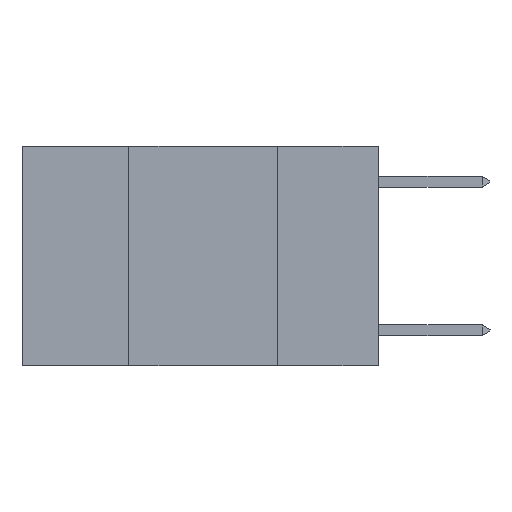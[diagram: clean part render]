
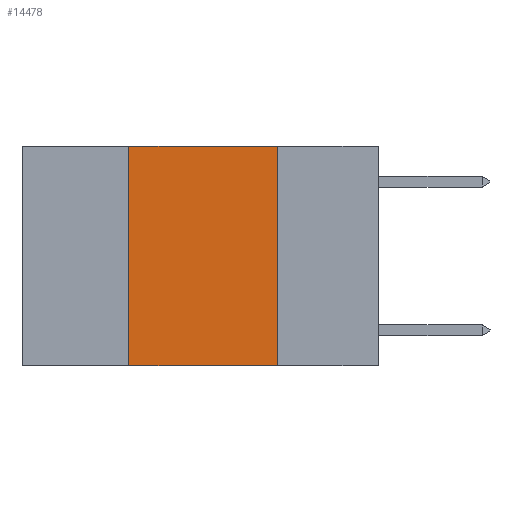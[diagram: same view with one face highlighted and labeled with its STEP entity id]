
A CAD part, left-side view. The second image highlights one B-rep face of the part: STEP entity #14478.
In plain terms, the highlighted planar face has unit normal (-1, 0, 0).
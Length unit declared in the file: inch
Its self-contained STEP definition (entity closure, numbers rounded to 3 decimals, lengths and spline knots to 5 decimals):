
#86 = PLANE ( 'NONE',  #13197 ) ;
#135 = DIRECTION ( 'NONE',  ( 0., 0., 1. ) ) ;
#991 = LINE ( 'NONE', #5284, #12926 ) ;
#1538 = CARTESIAN_POINT ( 'NONE',  ( 0., 0.17, -0.37 ) ) ;
#1664 = LINE ( 'NONE', #14514, #7647 ) ;
#2392 = DIRECTION ( 'NONE',  ( 0., 0., -1. ) ) ;
#2948 = DIRECTION ( 'NONE',  ( 0., 0., -1. ) ) ;
#4117 = VECTOR ( 'NONE', #7695, 39.37008 ) ;
#4476 = LINE ( 'NONE', #11189, #4117 ) ;
#5254 = EDGE_LOOP ( 'NONE', ( #14675, #10217, #8213, #11137 ) ) ;
#5284 = CARTESIAN_POINT ( 'NONE',  ( 0., 0.17, 0. ) ) ;
#5520 = VERTEX_POINT ( 'NONE', #14484 ) ;
#6291 = VERTEX_POINT ( 'NONE', #13786 ) ;
#7647 = VECTOR ( 'NONE', #13529, 39.37008 ) ;
#7695 = DIRECTION ( 'NONE',  ( 0., -1., 0. ) ) ;
#7949 = VERTEX_POINT ( 'NONE', #1538 ) ;
#8076 = VECTOR ( 'NONE', #135, 39.37008 ) ;
#8213 = ORIENTED_EDGE ( 'NONE', *, *, #12576, .F. ) ;
#8333 = CARTESIAN_POINT ( 'NONE',  ( 0., 0.6, 0. ) ) ;
#9514 = DIRECTION ( 'NONE',  ( 1., 0., 0. ) ) ;
#10217 = ORIENTED_EDGE ( 'NONE', *, *, #13520, .F. ) ;
#10666 = CARTESIAN_POINT ( 'NONE',  ( 0., 0.17, 0. ) ) ;
#11137 = ORIENTED_EDGE ( 'NONE', *, *, #14296, .T. ) ;
#11189 = CARTESIAN_POINT ( 'NONE',  ( 0., 0.6, 0. ) ) ;
#12576 = EDGE_CURVE ( 'NONE', #5520, #6291, #13914, .T. ) ;
#12578 = VERTEX_POINT ( 'NONE', #10666 ) ;
#12926 = VECTOR ( 'NONE', #2948, 39.37008 ) ;
#13197 = AXIS2_PLACEMENT_3D ( 'NONE', #8333, #9514, #2392 ) ;
#13514 = EDGE_CURVE ( 'NONE', #12578, #7949, #991, .T. ) ;
#13520 = EDGE_CURVE ( 'NONE', #6291, #12578, #4476, .T. ) ;
#13529 = DIRECTION ( 'NONE',  ( 0., -1., 0. ) ) ;
#13786 = CARTESIAN_POINT ( 'NONE',  ( 0., 0.42, 0. ) ) ;
#13849 = CARTESIAN_POINT ( 'NONE',  ( 0., 0.42, 0. ) ) ;
#13914 = LINE ( 'NONE', #13849, #8076 ) ;
#14015 = FACE_OUTER_BOUND ( 'NONE', #5254, .T. ) ;
#14296 = EDGE_CURVE ( 'NONE', #5520, #7949, #1664, .T. ) ;
#14478 = ADVANCED_FACE ( 'NONE', ( #14015 ), #86, .F. ) ;
#14484 = CARTESIAN_POINT ( 'NONE',  ( 0., 0.42, -0.37 ) ) ;
#14514 = CARTESIAN_POINT ( 'NONE',  ( 0., 0.6, -0.37 ) ) ;
#14675 = ORIENTED_EDGE ( 'NONE', *, *, #13514, .F. ) ;
